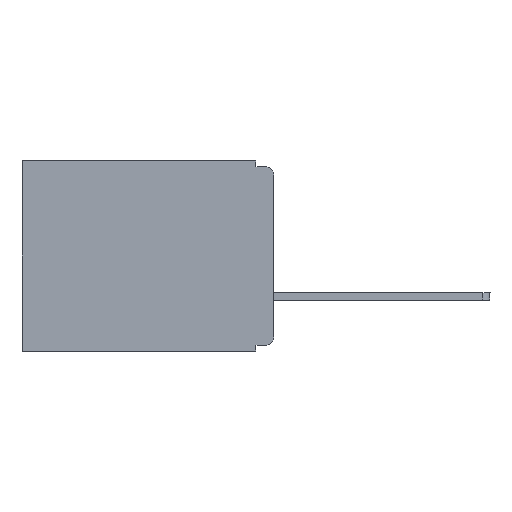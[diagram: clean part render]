
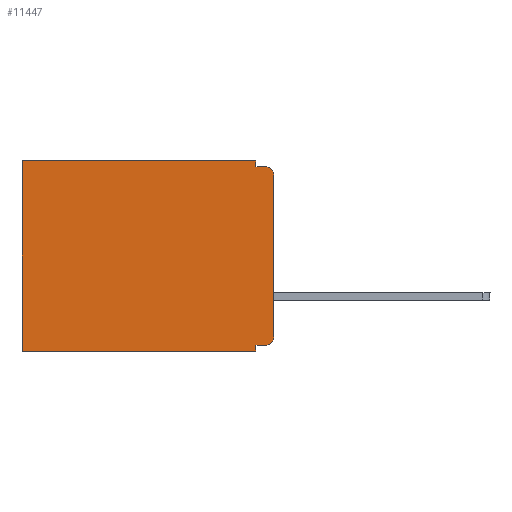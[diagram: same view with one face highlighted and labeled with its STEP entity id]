
A CAD part, left-side view. The second image highlights one B-rep face of the part: STEP entity #11447.
In plain terms, the highlighted planar face has unit normal (-1, 0, 0).
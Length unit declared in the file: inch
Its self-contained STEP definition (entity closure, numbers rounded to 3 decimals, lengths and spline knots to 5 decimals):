
#80 = VERTEX_POINT ( 'NONE', #12927 ) ;
#126 = EDGE_CURVE ( 'NONE', #11441, #9337, #1668, .T. ) ;
#327 = ORIENTED_EDGE ( 'NONE', *, *, #13529, .T. ) ;
#333 = VERTEX_POINT ( 'NONE', #11372 ) ;
#363 = EDGE_CURVE ( 'NONE', #1091, #9337, #4902, .T. ) ;
#461 = VECTOR ( 'NONE', #6615, 39.37008 ) ;
#584 = CARTESIAN_POINT ( 'NONE',  ( 0.3, 0.031, 0. ) ) ;
#922 = DIRECTION ( 'NONE',  ( 0., 0., -1. ) ) ;
#1091 = VERTEX_POINT ( 'NONE', #7985 ) ;
#1355 = EDGE_CURVE ( 'NONE', #14054, #13933, #8700, .T. ) ;
#1444 = CARTESIAN_POINT ( 'NONE',  ( 0.3, 0.031, 0. ) ) ;
#1465 = FACE_OUTER_BOUND ( 'NONE', #9178, .T. ) ;
#1668 = CIRCLE ( 'NONE', #9230, 0.015 ) ;
#2305 = ORIENTED_EDGE ( 'NONE', *, *, #6424, .T. ) ;
#2685 = DIRECTION ( 'NONE',  ( 0., 0., -1. ) ) ;
#2963 = CARTESIAN_POINT ( 'NONE',  ( 0.3, 0.437, -0.33 ) ) ;
#3229 = ORIENTED_EDGE ( 'NONE', *, *, #12103, .F. ) ;
#3342 = PLANE ( 'NONE',  #7522 ) ;
#3377 = VECTOR ( 'NONE', #13288, 39.37008 ) ;
#3525 = CARTESIAN_POINT ( 'NONE',  ( 0.3, 0.015, -0.305 ) ) ;
#3529 = EDGE_CURVE ( 'NONE', #1091, #11747, #15096, .T. ) ;
#3730 = DIRECTION ( 'NONE',  ( 0., 0., -1. ) ) ;
#3899 = CARTESIAN_POINT ( 'NONE',  ( 0.3, 0.015, -0.025 ) ) ;
#4001 = DIRECTION ( 'NONE',  ( 0., 0., -1. ) ) ;
#4121 = DIRECTION ( 'NONE',  ( 0., -1., 0. ) ) ;
#4166 = CARTESIAN_POINT ( 'NONE',  ( 0.3, 0., -0.305 ) ) ;
#4902 = LINE ( 'NONE', #8964, #11772 ) ;
#5352 = DIRECTION ( 'NONE',  ( 0., 0., -1. ) ) ;
#5464 = LINE ( 'NONE', #11729, #12523 ) ;
#5893 = ORIENTED_EDGE ( 'NONE', *, *, #7159, .F. ) ;
#6087 = CARTESIAN_POINT ( 'NONE',  ( 0.3, 0., -0.32 ) ) ;
#6105 = CARTESIAN_POINT ( 'NONE',  ( 0.3, 0., -0.33 ) ) ;
#6424 = EDGE_CURVE ( 'NONE', #14054, #80, #8746, .T. ) ;
#6615 = DIRECTION ( 'NONE',  ( 0., 0., -1. ) ) ;
#7159 = EDGE_CURVE ( 'NONE', #11441, #14421, #9479, .T. ) ;
#7271 = ORIENTED_EDGE ( 'NONE', *, *, #8842, .F. ) ;
#7334 = LINE ( 'NONE', #11577, #461 ) ;
#7522 = AXIS2_PLACEMENT_3D ( 'NONE', #6105, #12141, #10905 ) ;
#7829 = EDGE_CURVE ( 'NONE', #13933, #11747, #14389, .T. ) ;
#7831 = CARTESIAN_POINT ( 'NONE',  ( 0.3, 0.031, -0.01 ) ) ;
#7968 = VERTEX_POINT ( 'NONE', #10745 ) ;
#7985 = CARTESIAN_POINT ( 'NONE',  ( 0.3, 0., -0.025 ) ) ;
#8047 = DIRECTION ( 'NONE',  ( 0., 1., 0. ) ) ;
#8183 = DIRECTION ( 'NONE',  ( 0., 1., 0. ) ) ;
#8420 = ORIENTED_EDGE ( 'NONE', *, *, #1355, .F. ) ;
#8700 = LINE ( 'NONE', #1444, #13073 ) ;
#8746 = LINE ( 'NONE', #9447, #15000 ) ;
#8842 = EDGE_CURVE ( 'NONE', #14421, #333, #7334, .T. ) ;
#8895 = ORIENTED_EDGE ( 'NONE', *, *, #3529, .T. ) ;
#8953 = ORIENTED_EDGE ( 'NONE', *, *, #363, .F. ) ;
#8964 = CARTESIAN_POINT ( 'NONE',  ( 0.3, 0., -0.33 ) ) ;
#9178 = EDGE_LOOP ( 'NONE', ( #8953, #8895, #10325, #8420, #2305, #327, #3229, #7271, #5893, #15587 ) ) ;
#9230 = AXIS2_PLACEMENT_3D ( 'NONE', #3525, #13195, #922 ) ;
#9337 = VERTEX_POINT ( 'NONE', #4166 ) ;
#9447 = CARTESIAN_POINT ( 'NONE',  ( 0.3, 0., 0. ) ) ;
#9479 = LINE ( 'NONE', #6087, #3377 ) ;
#10325 = ORIENTED_EDGE ( 'NONE', *, *, #7829, .F. ) ;
#10689 = CARTESIAN_POINT ( 'NONE',  ( 0.3, 0.015, -0.32 ) ) ;
#10745 = CARTESIAN_POINT ( 'NONE',  ( 0.3, 0.437, -0.33 ) ) ;
#10905 = DIRECTION ( 'NONE',  ( 0., 0., -1. ) ) ;
#11181 = VECTOR ( 'NONE', #4121, 39.37008 ) ;
#11372 = CARTESIAN_POINT ( 'NONE',  ( 0.3, 0.031, -0.33 ) ) ;
#11441 = VERTEX_POINT ( 'NONE', #10689 ) ;
#11447 = ADVANCED_FACE ( 'NONE', ( #1465 ), #3342, .F. ) ;
#11535 = CARTESIAN_POINT ( 'NONE',  ( 0.3, 0.031, -0.32 ) ) ;
#11577 = CARTESIAN_POINT ( 'NONE',  ( 0.3, 0.031, -0.33 ) ) ;
#11721 = VECTOR ( 'NONE', #5352, 39.37008 ) ;
#11729 = CARTESIAN_POINT ( 'NONE',  ( 0.3, 0., -0.33 ) ) ;
#11747 = VERTEX_POINT ( 'NONE', #12024 ) ;
#11772 = VECTOR ( 'NONE', #2685, 39.37008 ) ;
#11904 = LINE ( 'NONE', #2963, #11721 ) ;
#12024 = CARTESIAN_POINT ( 'NONE',  ( 0.3, 0.015, -0.01 ) ) ;
#12103 = EDGE_CURVE ( 'NONE', #333, #7968, #5464, .T. ) ;
#12141 = DIRECTION ( 'NONE',  ( 1., 0., 0. ) ) ;
#12523 = VECTOR ( 'NONE', #8183, 39.37008 ) ;
#12927 = CARTESIAN_POINT ( 'NONE',  ( 0.3, 0.437, 0. ) ) ;
#13073 = VECTOR ( 'NONE', #3730, 39.37008 ) ;
#13195 = DIRECTION ( 'NONE',  ( -1., 0., 0. ) ) ;
#13288 = DIRECTION ( 'NONE',  ( 0., 1., 0. ) ) ;
#13529 = EDGE_CURVE ( 'NONE', #80, #7968, #11904, .T. ) ;
#13613 = DIRECTION ( 'NONE',  ( -1., 0., 0. ) ) ;
#13933 = VERTEX_POINT ( 'NONE', #7831 ) ;
#13988 = CARTESIAN_POINT ( 'NONE',  ( 0.3, 0., -0.01 ) ) ;
#14054 = VERTEX_POINT ( 'NONE', #584 ) ;
#14174 = AXIS2_PLACEMENT_3D ( 'NONE', #3899, #13613, #4001 ) ;
#14389 = LINE ( 'NONE', #13988, #11181 ) ;
#14421 = VERTEX_POINT ( 'NONE', #11535 ) ;
#15000 = VECTOR ( 'NONE', #8047, 39.37008 ) ;
#15096 = CIRCLE ( 'NONE', #14174, 0.015 ) ;
#15587 = ORIENTED_EDGE ( 'NONE', *, *, #126, .T. ) ;
